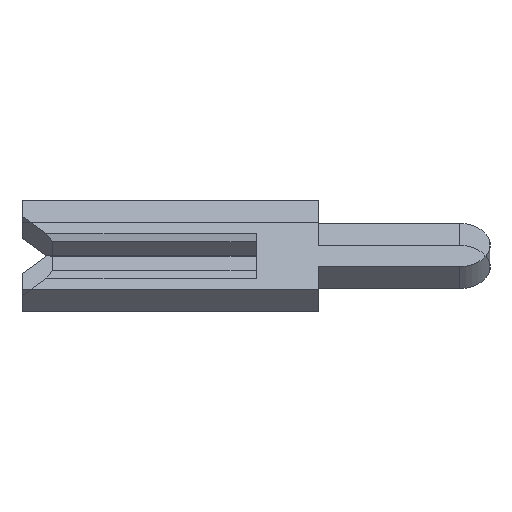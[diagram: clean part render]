
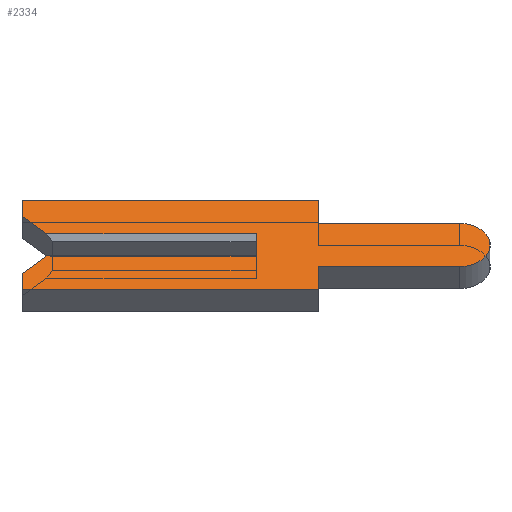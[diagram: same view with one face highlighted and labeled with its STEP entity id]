
A CAD part, left-side view. The second image highlights one B-rep face of the part: STEP entity #2334.
In plain terms, the highlighted face is planar.
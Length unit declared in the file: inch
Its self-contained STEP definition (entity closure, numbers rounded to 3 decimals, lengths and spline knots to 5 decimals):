
#2 = CARTESIAN_POINT ( 'NONE',  ( -0.01, -0.04, 0.04 ) ) ;
#24 = EDGE_CURVE ( 'NONE', #2188, #770, #2388, .T. ) ;
#71 = CARTESIAN_POINT ( 'NONE',  ( -0.01, -0.1305, 0. ) ) ;
#88 = VERTEX_POINT ( 'NONE', #982 ) ;
#101 = DIRECTION ( 'NONE',  ( 0., -1., 0. ) ) ;
#134 = CARTESIAN_POINT ( 'NONE',  ( -0.01, -0.04, -0.0195 ) ) ;
#167 = ORIENTED_EDGE ( 'NONE', *, *, #185, .F. ) ;
#172 = VERTEX_POINT ( 'NONE', #1594 ) ;
#185 = EDGE_CURVE ( 'NONE', #88, #172, #268, .T. ) ;
#189 = VERTEX_POINT ( 'NONE', #1218 ) ;
#228 = EDGE_CURVE ( 'NONE', #348, #2027, #1195, .T. ) ;
#268 = LINE ( 'NONE', #2382, #906 ) ;
#272 = VECTOR ( 'NONE', #1525, 39.37008 ) ;
#293 = CARTESIAN_POINT ( 'NONE',  ( -0.01, 0.15, 0.04 ) ) ;
#298 = VECTOR ( 'NONE', #1181, 39.37008 ) ;
#300 = EDGE_CURVE ( 'NONE', #777, #1877, #1080, .T. ) ;
#305 = CIRCLE ( 'NONE', #511, 0.0195 ) ;
#316 = VECTOR ( 'NONE', #2363, 39.37008 ) ;
#348 = VERTEX_POINT ( 'NONE', #519 ) ;
#374 = CARTESIAN_POINT ( 'NONE',  ( -0.01, -0.04, 0.0195 ) ) ;
#377 = LINE ( 'NONE', #479, #1014 ) ;
#384 = ORIENTED_EDGE ( 'NONE', *, *, #2387, .F. ) ;
#385 = EDGE_CURVE ( 'NONE', #1661, #777, #1537, .T. ) ;
#418 = LINE ( 'NONE', #946, #1381 ) ;
#437 = LINE ( 'NONE', #1214, #1082 ) ;
#448 = CARTESIAN_POINT ( 'NONE',  ( -0.01, 0.1305, 0.0065 ) ) ;
#455 = DIRECTION ( 'NONE',  ( 0., 0., -1. ) ) ;
#479 = CARTESIAN_POINT ( 'NONE',  ( -0.01, 0.15, 0.026 ) ) ;
#508 = VECTOR ( 'NONE', #1885, 39.37008 ) ;
#511 = AXIS2_PLACEMENT_3D ( 'NONE', #535, #1124, #2123 ) ;
#519 = CARTESIAN_POINT ( 'NONE',  ( -0.01, 0.134, 0.01 ) ) ;
#535 = CARTESIAN_POINT ( 'NONE',  ( -0.01, -0.1305, 0. ) ) ;
#542 = EDGE_CURVE ( 'NONE', #189, #88, #2451, .T. ) ;
#557 = VECTOR ( 'NONE', #1803, 39.37008 ) ;
#570 = ORIENTED_EDGE ( 'NONE', *, *, #934, .F. ) ;
#598 = DIRECTION ( 'NONE',  ( 0., 0., 1. ) ) ;
#620 = VECTOR ( 'NONE', #101, 39.37008 ) ;
#635 = ORIENTED_EDGE ( 'NONE', *, *, #2187, .F. ) ;
#636 = CARTESIAN_POINT ( 'NONE',  ( -0.01, 0.15, 0.04 ) ) ;
#652 = DIRECTION ( 'NONE',  ( 0., 0., 1. ) ) ;
#740 = VERTEX_POINT ( 'NONE', #1872 ) ;
#770 = VERTEX_POINT ( 'NONE', #1419 ) ;
#777 = VERTEX_POINT ( 'NONE', #2268 ) ;
#783 = ORIENTED_EDGE ( 'NONE', *, *, #542, .F. ) ;
#784 = ORIENTED_EDGE ( 'NONE', *, *, #385, .F. ) ;
#785 = LINE ( 'NONE', #1698, #272 ) ;
#791 = CARTESIAN_POINT ( 'NONE',  ( -0.01, -0.1305, 0.0195 ) ) ;
#816 = VECTOR ( 'NONE', #2474, 39.37008 ) ;
#834 = LINE ( 'NONE', #2, #316 ) ;
#906 = VECTOR ( 'NONE', #598, 39.37008 ) ;
#934 = EDGE_CURVE ( 'NONE', #1551, #1661, #305, .T. ) ;
#945 = LINE ( 'NONE', #374, #1884 ) ;
#946 = CARTESIAN_POINT ( 'NONE',  ( -0.01, 0.15, -0.04 ) ) ;
#982 = CARTESIAN_POINT ( 'NONE',  ( -0.01, 0., -0.01 ) ) ;
#1014 = VECTOR ( 'NONE', #652, 39.37008 ) ;
#1018 = VERTEX_POINT ( 'NONE', #1748 ) ;
#1072 = EDGE_CURVE ( 'NONE', #1877, #2188, #418, .T. ) ;
#1080 = LINE ( 'NONE', #2238, #1198 ) ;
#1082 = VECTOR ( 'NONE', #1398, 39.37008 ) ;
#1108 = EDGE_CURVE ( 'NONE', #348, #172, #785, .T. ) ;
#1124 = DIRECTION ( 'NONE',  ( 1., 0., 0. ) ) ;
#1143 = DIRECTION ( 'NONE',  ( 0., 1., 0. ) ) ;
#1161 = AXIS2_PLACEMENT_3D ( 'NONE', #71, #1268, #455 ) ;
#1181 = DIRECTION ( 'NONE',  ( 0., 0., 1. ) ) ;
#1195 = LINE ( 'NONE', #448, #557 ) ;
#1198 = VECTOR ( 'NONE', #2088, 39.37008 ) ;
#1201 = CARTESIAN_POINT ( 'NONE',  ( -0.01, 0.15, 0.026 ) ) ;
#1214 = CARTESIAN_POINT ( 'NONE',  ( -0.01, 0.1305, -0.0065 ) ) ;
#1218 = CARTESIAN_POINT ( 'NONE',  ( -0.01, 0.134, -0.01 ) ) ;
#1268 = DIRECTION ( 'NONE',  ( 1., 0., 0. ) ) ;
#1381 = VECTOR ( 'NONE', #1143, 39.37008 ) ;
#1390 = CARTESIAN_POINT ( 'NONE',  ( -0.01, -0.04, -0.04 ) ) ;
#1398 = DIRECTION ( 'NONE',  ( 0., -0.707, 0.707 ) ) ;
#1419 = CARTESIAN_POINT ( 'NONE',  ( -0.01, 0.15, -0.026 ) ) ;
#1515 = EDGE_CURVE ( 'NONE', #740, #1551, #945, .T. ) ;
#1525 = DIRECTION ( 'NONE',  ( 0., -1., 0. ) ) ;
#1537 = LINE ( 'NONE', #134, #508 ) ;
#1551 = VERTEX_POINT ( 'NONE', #791 ) ;
#1594 = CARTESIAN_POINT ( 'NONE',  ( -0.01, 0., 0.01 ) ) ;
#1649 = EDGE_LOOP ( 'NONE', ( #1973, #167, #783, #635, #2209, #1843, #1928, #784, #570, #2285, #1904, #384, #1925, #2223 ) ) ;
#1661 = VERTEX_POINT ( 'NONE', #1965 ) ;
#1698 = CARTESIAN_POINT ( 'NONE',  ( -0.01, 0.15, 0.01 ) ) ;
#1722 = CARTESIAN_POINT ( 'NONE',  ( -0.01, 0.15, -0.026 ) ) ;
#1736 = EDGE_CURVE ( 'NONE', #1018, #740, #834, .T. ) ;
#1748 = CARTESIAN_POINT ( 'NONE',  ( -0.01, -0.04, 0.04 ) ) ;
#1803 = DIRECTION ( 'NONE',  ( 0., 0.707, 0.707 ) ) ;
#1828 = CARTESIAN_POINT ( 'NONE',  ( -0.01, -0.1305, -0.01 ) ) ;
#1839 = FACE_OUTER_BOUND ( 'NONE', #1649, .T. ) ;
#1843 = ORIENTED_EDGE ( 'NONE', *, *, #1072, .F. ) ;
#1872 = CARTESIAN_POINT ( 'NONE',  ( -0.01, -0.04, 0.0195 ) ) ;
#1877 = VERTEX_POINT ( 'NONE', #1390 ) ;
#1884 = VECTOR ( 'NONE', #1974, 39.37008 ) ;
#1885 = DIRECTION ( 'NONE',  ( 0., 1., 0. ) ) ;
#1904 = ORIENTED_EDGE ( 'NONE', *, *, #1736, .F. ) ;
#1925 = ORIENTED_EDGE ( 'NONE', *, *, #2443, .F. ) ;
#1928 = ORIENTED_EDGE ( 'NONE', *, *, #300, .F. ) ;
#1965 = CARTESIAN_POINT ( 'NONE',  ( -0.01, -0.1305, -0.0195 ) ) ;
#1973 = ORIENTED_EDGE ( 'NONE', *, *, #1108, .T. ) ;
#1974 = DIRECTION ( 'NONE',  ( 0., -1., 0. ) ) ;
#1981 = CARTESIAN_POINT ( 'NONE',  ( -0.01, 0.15, -0.04 ) ) ;
#2027 = VERTEX_POINT ( 'NONE', #1201 ) ;
#2088 = DIRECTION ( 'NONE',  ( 0., 0., -1. ) ) ;
#2094 = LINE ( 'NONE', #293, #620 ) ;
#2123 = DIRECTION ( 'NONE',  ( 0., 0., -1. ) ) ;
#2187 = EDGE_CURVE ( 'NONE', #770, #189, #437, .T. ) ;
#2188 = VERTEX_POINT ( 'NONE', #1981 ) ;
#2209 = ORIENTED_EDGE ( 'NONE', *, *, #24, .F. ) ;
#2223 = ORIENTED_EDGE ( 'NONE', *, *, #228, .F. ) ;
#2225 = PLANE ( 'NONE',  #1161 ) ;
#2232 = VERTEX_POINT ( 'NONE', #636 ) ;
#2238 = CARTESIAN_POINT ( 'NONE',  ( -0.01, -0.04, -0.04 ) ) ;
#2268 = CARTESIAN_POINT ( 'NONE',  ( -0.01, -0.04, -0.0195 ) ) ;
#2285 = ORIENTED_EDGE ( 'NONE', *, *, #1515, .F. ) ;
#2334 = ADVANCED_FACE ( 'NONE', ( #1839 ), #2225, .F. ) ;
#2363 = DIRECTION ( 'NONE',  ( 0., 0., -1. ) ) ;
#2382 = CARTESIAN_POINT ( 'NONE',  ( -0.01, 0., 0.0065 ) ) ;
#2387 = EDGE_CURVE ( 'NONE', #2232, #1018, #2094, .T. ) ;
#2388 = LINE ( 'NONE', #1722, #298 ) ;
#2443 = EDGE_CURVE ( 'NONE', #2027, #2232, #377, .T. ) ;
#2451 = LINE ( 'NONE', #1828, #816 ) ;
#2474 = DIRECTION ( 'NONE',  ( 0., -1., 0. ) ) ;
